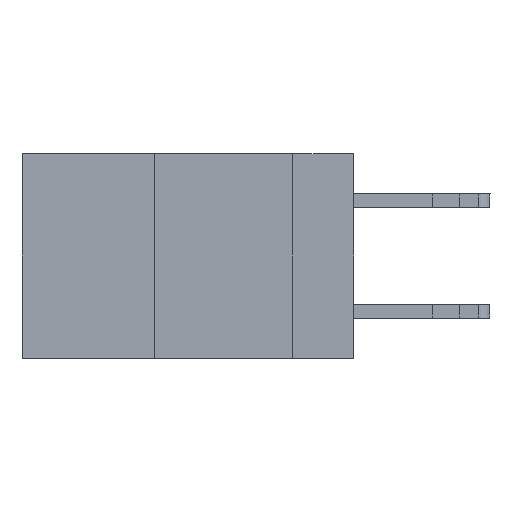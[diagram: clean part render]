
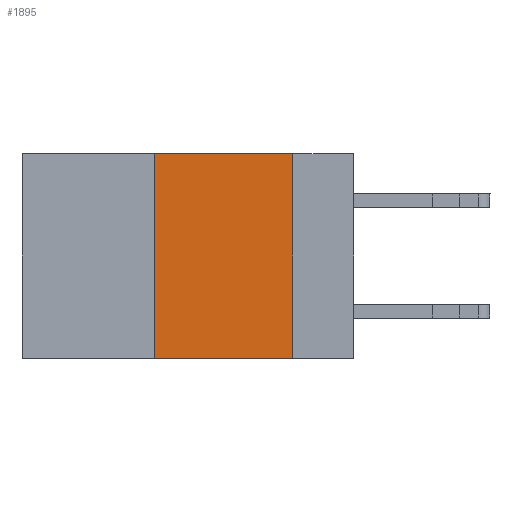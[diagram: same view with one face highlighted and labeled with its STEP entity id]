
A CAD part, left-side view. The second image highlights one B-rep face of the part: STEP entity #1895.
In plain terms, the highlighted planar face has unit normal (-1, 0, 0).
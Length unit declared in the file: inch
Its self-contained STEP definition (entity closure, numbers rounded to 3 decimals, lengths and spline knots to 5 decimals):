
#161 = EDGE_CURVE ( 'NONE', #19257, #14186, #4246, .T. ) ;
#649 = DIRECTION ( 'NONE',  ( 0., 0., 1. ) ) ;
#1683 = CARTESIAN_POINT ( 'NONE',  ( 0., 0.11, 0. ) ) ;
#1895 = ADVANCED_FACE ( 'NONE', ( #13061 ), #25462, .F. ) ;
#2074 = VECTOR ( 'NONE', #3930, 39.37008 ) ;
#2317 = VECTOR ( 'NONE', #8450, 39.37008 ) ;
#3541 = VERTEX_POINT ( 'NONE', #14142 ) ;
#3930 = DIRECTION ( 'NONE',  ( 0., 0., -1. ) ) ;
#4246 = LINE ( 'NONE', #1683, #2074 ) ;
#6115 = EDGE_CURVE ( 'NONE', #22875, #14186, #25815, .T. ) ;
#6703 = CARTESIAN_POINT ( 'NONE',  ( 0., 0.11, -0.37 ) ) ;
#7322 = EDGE_CURVE ( 'NONE', #22875, #3541, #12182, .T. ) ;
#8450 = DIRECTION ( 'NONE',  ( 0., -1., 0. ) ) ;
#10395 = LINE ( 'NONE', #13274, #29654 ) ;
#10504 = CARTESIAN_POINT ( 'NONE',  ( 0., 0.36, -0.37 ) ) ;
#12182 = LINE ( 'NONE', #22504, #12443 ) ;
#12443 = VECTOR ( 'NONE', #649, 39.37008 ) ;
#13061 = FACE_OUTER_BOUND ( 'NONE', #28107, .T. ) ;
#13274 = CARTESIAN_POINT ( 'NONE',  ( 0., 0.6, 0. ) ) ;
#14142 = CARTESIAN_POINT ( 'NONE',  ( 0., 0.36, 0. ) ) ;
#14186 = VERTEX_POINT ( 'NONE', #6703 ) ;
#15436 = DIRECTION ( 'NONE',  ( 0., 0., -1. ) ) ;
#15498 = ORIENTED_EDGE ( 'NONE', *, *, #161, .F. ) ;
#17569 = DIRECTION ( 'NONE',  ( 0., -1., 0. ) ) ;
#18337 = EDGE_CURVE ( 'NONE', #3541, #19257, #10395, .T. ) ;
#19257 = VERTEX_POINT ( 'NONE', #20761 ) ;
#20761 = CARTESIAN_POINT ( 'NONE',  ( 0., 0.11, 0. ) ) ;
#21020 = ORIENTED_EDGE ( 'NONE', *, *, #18337, .F. ) ;
#21670 = AXIS2_PLACEMENT_3D ( 'NONE', #25623, #30565, #15436 ) ;
#22504 = CARTESIAN_POINT ( 'NONE',  ( 0., 0.36, 0. ) ) ;
#22875 = VERTEX_POINT ( 'NONE', #10504 ) ;
#23100 = ORIENTED_EDGE ( 'NONE', *, *, #6115, .T. ) ;
#25462 = PLANE ( 'NONE',  #21670 ) ;
#25623 = CARTESIAN_POINT ( 'NONE',  ( 0., 0.6, 0. ) ) ;
#25815 = LINE ( 'NONE', #28199, #2317 ) ;
#27713 = ORIENTED_EDGE ( 'NONE', *, *, #7322, .F. ) ;
#28107 = EDGE_LOOP ( 'NONE', ( #15498, #21020, #27713, #23100 ) ) ;
#28199 = CARTESIAN_POINT ( 'NONE',  ( 0., 0.6, -0.37 ) ) ;
#29654 = VECTOR ( 'NONE', #17569, 39.37008 ) ;
#30565 = DIRECTION ( 'NONE',  ( 1., 0., 0. ) ) ;
